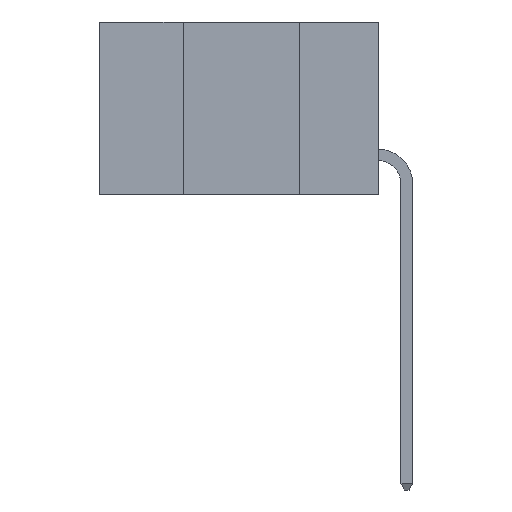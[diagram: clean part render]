
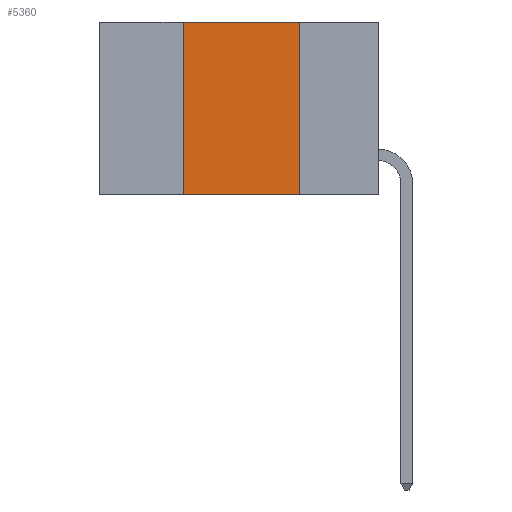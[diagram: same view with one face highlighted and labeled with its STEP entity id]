
A CAD part, left-side view. The second image highlights one B-rep face of the part: STEP entity #5360.
In plain terms, the highlighted planar face has unit normal (-1, 0, 0).
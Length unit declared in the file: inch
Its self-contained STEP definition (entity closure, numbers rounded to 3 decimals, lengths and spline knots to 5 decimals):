
#175 = EDGE_CURVE ( 'NONE', #15649, #10778, #15435, .T. ) ;
#265 = ORIENTED_EDGE ( 'NONE', *, *, #1144, .F. ) ;
#755 = VERTEX_POINT ( 'NONE', #11068 ) ;
#1144 = EDGE_CURVE ( 'NONE', #10778, #7438, #17616, .T. ) ;
#1549 = CARTESIAN_POINT ( 'NONE',  ( 0., 0.17, -0.37 ) ) ;
#1558 = VECTOR ( 'NONE', #6868, 39.37008 ) ;
#1852 = DIRECTION ( 'NONE',  ( 0., 0., -1. ) ) ;
#2379 = DIRECTION ( 'NONE',  ( 0., 0., -1. ) ) ;
#3444 = EDGE_LOOP ( 'NONE', ( #265, #9156, #15992, #4573 ) ) ;
#4573 = ORIENTED_EDGE ( 'NONE', *, *, #16400, .T. ) ;
#5130 = CARTESIAN_POINT ( 'NONE',  ( 0., 0.17, -0.37 ) ) ;
#5360 = ADVANCED_FACE ( 'NONE', ( #7129 ), #6097, .F. ) ;
#6097 = PLANE ( 'NONE',  #17743 ) ;
#6868 = DIRECTION ( 'NONE',  ( 0., 0., 1. ) ) ;
#7129 = FACE_OUTER_BOUND ( 'NONE', #3444, .T. ) ;
#7438 = VERTEX_POINT ( 'NONE', #5130 ) ;
#7497 = CARTESIAN_POINT ( 'NONE',  ( 0., 0.6, 0. ) ) ;
#8656 = LINE ( 'NONE', #13855, #1558 ) ;
#8691 = VECTOR ( 'NONE', #17144, 39.37008 ) ;
#9156 = ORIENTED_EDGE ( 'NONE', *, *, #175, .F. ) ;
#10321 = DIRECTION ( 'NONE',  ( 1., 0., 0. ) ) ;
#10506 = VECTOR ( 'NONE', #2379, 39.37008 ) ;
#10778 = VERTEX_POINT ( 'NONE', #17404 ) ;
#11068 = CARTESIAN_POINT ( 'NONE',  ( 0., 0.42, -0.37 ) ) ;
#11784 = CARTESIAN_POINT ( 'NONE',  ( 0., 0.6, -0.37 ) ) ;
#11848 = VECTOR ( 'NONE', #16048, 39.37008 ) ;
#12425 = LINE ( 'NONE', #11784, #8691 ) ;
#13855 = CARTESIAN_POINT ( 'NONE',  ( 0., 0.42, -0.37 ) ) ;
#15435 = LINE ( 'NONE', #17523, #11848 ) ;
#15649 = VERTEX_POINT ( 'NONE', #15691 ) ;
#15691 = CARTESIAN_POINT ( 'NONE',  ( 0., 0.42, 0. ) ) ;
#15992 = ORIENTED_EDGE ( 'NONE', *, *, #17260, .F. ) ;
#16048 = DIRECTION ( 'NONE',  ( 0., -1., 0. ) ) ;
#16400 = EDGE_CURVE ( 'NONE', #755, #7438, #12425, .T. ) ;
#17144 = DIRECTION ( 'NONE',  ( 0., -1., 0. ) ) ;
#17260 = EDGE_CURVE ( 'NONE', #755, #15649, #8656, .T. ) ;
#17404 = CARTESIAN_POINT ( 'NONE',  ( 0., 0.17, 0. ) ) ;
#17523 = CARTESIAN_POINT ( 'NONE',  ( 0., 0.6, 0. ) ) ;
#17616 = LINE ( 'NONE', #1549, #10506 ) ;
#17743 = AXIS2_PLACEMENT_3D ( 'NONE', #7497, #10321, #1852 ) ;
